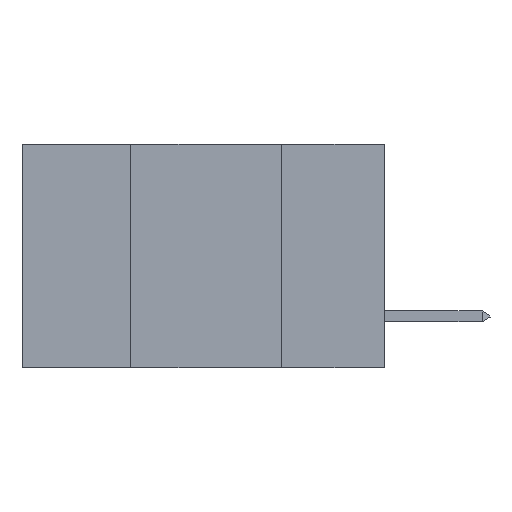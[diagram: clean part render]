
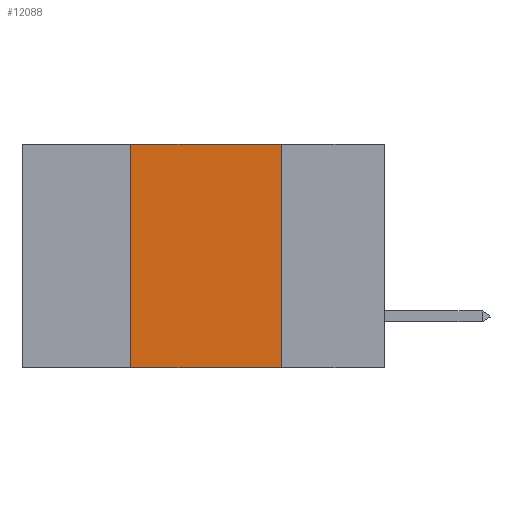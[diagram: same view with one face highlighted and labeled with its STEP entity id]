
A CAD part, left-side view. The second image highlights one B-rep face of the part: STEP entity #12088.
In plain terms, the highlighted planar face has unit normal (-1, 0, 0).
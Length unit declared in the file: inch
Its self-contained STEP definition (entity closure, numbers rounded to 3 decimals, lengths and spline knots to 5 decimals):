
#307 = DIRECTION ( 'NONE',  ( 0., -1., 0. ) ) ;
#339 = VERTEX_POINT ( 'NONE', #14222 ) ;
#852 = VERTEX_POINT ( 'NONE', #13241 ) ;
#1271 = LINE ( 'NONE', #5100, #1643 ) ;
#1393 = DIRECTION ( 'NONE',  ( 0., 0., -1. ) ) ;
#1643 = VECTOR ( 'NONE', #12905, 39.37008 ) ;
#1726 = CARTESIAN_POINT ( 'NONE',  ( 0., 0.17, 0. ) ) ;
#2245 = LINE ( 'NONE', #12449, #5223 ) ;
#2344 = ORIENTED_EDGE ( 'NONE', *, *, #7080, .F. ) ;
#3032 = VERTEX_POINT ( 'NONE', #1726 ) ;
#3249 = EDGE_CURVE ( 'NONE', #852, #3032, #2245, .T. ) ;
#3263 = FACE_OUTER_BOUND ( 'NONE', #7242, .T. ) ;
#4668 = PLANE ( 'NONE',  #8055 ) ;
#4794 = CARTESIAN_POINT ( 'NONE',  ( 0., 0.6, -0.37 ) ) ;
#4848 = EDGE_CURVE ( 'NONE', #10157, #852, #1271, .T. ) ;
#5100 = CARTESIAN_POINT ( 'NONE',  ( 0., 0.42, 0. ) ) ;
#5223 = VECTOR ( 'NONE', #307, 39.37008 ) ;
#5902 = ORIENTED_EDGE ( 'NONE', *, *, #5994, .T. ) ;
#5990 = LINE ( 'NONE', #4794, #7570 ) ;
#5994 = EDGE_CURVE ( 'NONE', #10157, #339, #5990, .T. ) ;
#6050 = CARTESIAN_POINT ( 'NONE',  ( 0., 0.17, 0. ) ) ;
#7080 = EDGE_CURVE ( 'NONE', #3032, #339, #10156, .T. ) ;
#7242 = EDGE_LOOP ( 'NONE', ( #2344, #7506, #13178, #5902 ) ) ;
#7370 = CARTESIAN_POINT ( 'NONE',  ( 0., 0.42, -0.37 ) ) ;
#7506 = ORIENTED_EDGE ( 'NONE', *, *, #3249, .F. ) ;
#7570 = VECTOR ( 'NONE', #12551, 39.37008 ) ;
#8055 = AXIS2_PLACEMENT_3D ( 'NONE', #10340, #12574, #9452 ) ;
#9452 = DIRECTION ( 'NONE',  ( 0., 0., -1. ) ) ;
#10156 = LINE ( 'NONE', #6050, #11705 ) ;
#10157 = VERTEX_POINT ( 'NONE', #7370 ) ;
#10340 = CARTESIAN_POINT ( 'NONE',  ( 0., 0.6, 0. ) ) ;
#11705 = VECTOR ( 'NONE', #1393, 39.37008 ) ;
#12088 = ADVANCED_FACE ( 'NONE', ( #3263 ), #4668, .F. ) ;
#12449 = CARTESIAN_POINT ( 'NONE',  ( 0., 0.6, 0. ) ) ;
#12551 = DIRECTION ( 'NONE',  ( 0., -1., 0. ) ) ;
#12574 = DIRECTION ( 'NONE',  ( 1., 0., 0. ) ) ;
#12905 = DIRECTION ( 'NONE',  ( 0., 0., 1. ) ) ;
#13178 = ORIENTED_EDGE ( 'NONE', *, *, #4848, .F. ) ;
#13241 = CARTESIAN_POINT ( 'NONE',  ( 0., 0.42, 0. ) ) ;
#14222 = CARTESIAN_POINT ( 'NONE',  ( 0., 0.17, -0.37 ) ) ;
